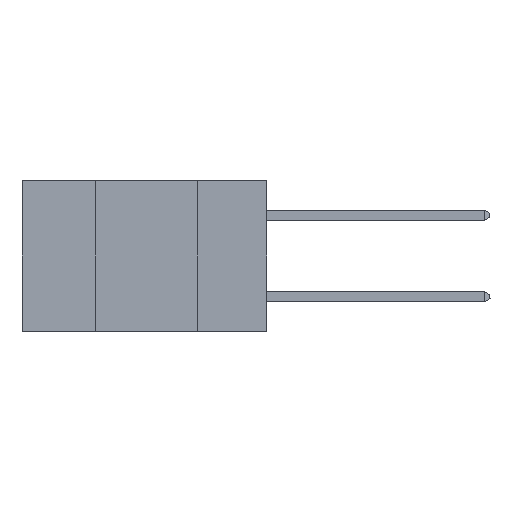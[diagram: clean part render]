
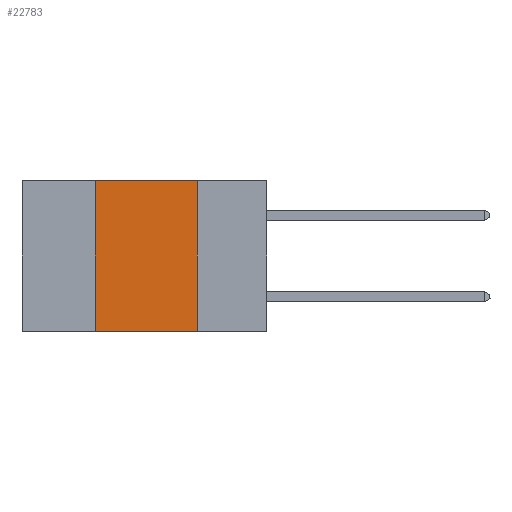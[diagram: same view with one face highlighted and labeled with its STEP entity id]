
A CAD part, left-side view. The second image highlights one B-rep face of the part: STEP entity #22783.
In plain terms, the highlighted planar face has unit normal (-1, 0, 0).
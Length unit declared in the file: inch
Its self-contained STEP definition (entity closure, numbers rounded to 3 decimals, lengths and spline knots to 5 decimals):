
#931 = VECTOR ( 'NONE', #15726, 39.37008 ) ;
#1160 = CARTESIAN_POINT ( 'NONE',  ( 0., 0.6, 0. ) ) ;
#2060 = LINE ( 'NONE', #25381, #29526 ) ;
#2293 = AXIS2_PLACEMENT_3D ( 'NONE', #1160, #17286, #24506 ) ;
#3103 = ORIENTED_EDGE ( 'NONE', *, *, #6593, .F. ) ;
#3889 = VERTEX_POINT ( 'NONE', #20650 ) ;
#4140 = CARTESIAN_POINT ( 'NONE',  ( 0., 0.42, 0. ) ) ;
#5482 = ORIENTED_EDGE ( 'NONE', *, *, #19721, .F. ) ;
#6108 = DIRECTION ( 'NONE',  ( 0., 0., -1. ) ) ;
#6310 = CARTESIAN_POINT ( 'NONE',  ( 0., 0.17, 0. ) ) ;
#6593 = EDGE_CURVE ( 'NONE', #18801, #10510, #7084, .T. ) ;
#7084 = LINE ( 'NONE', #4140, #931 ) ;
#7153 = CARTESIAN_POINT ( 'NONE',  ( 0., 0.42, -0.37 ) ) ;
#7213 = VECTOR ( 'NONE', #6108, 39.37008 ) ;
#10195 = ORIENTED_EDGE ( 'NONE', *, *, #24484, .T. ) ;
#10510 = VERTEX_POINT ( 'NONE', #27622 ) ;
#11272 = EDGE_LOOP ( 'NONE', ( #5482, #27780, #3103, #10195 ) ) ;
#11521 = DIRECTION ( 'NONE',  ( 0., -1., 0. ) ) ;
#14972 = PLANE ( 'NONE',  #2293 ) ;
#15726 = DIRECTION ( 'NONE',  ( 0., 0., 1. ) ) ;
#16009 = LINE ( 'NONE', #28918, #25049 ) ;
#17286 = DIRECTION ( 'NONE',  ( 1., 0., 0. ) ) ;
#18801 = VERTEX_POINT ( 'NONE', #7153 ) ;
#19678 = EDGE_CURVE ( 'NONE', #10510, #20355, #16009, .T. ) ;
#19721 = EDGE_CURVE ( 'NONE', #20355, #3889, #24591, .T. ) ;
#20355 = VERTEX_POINT ( 'NONE', #20448 ) ;
#20448 = CARTESIAN_POINT ( 'NONE',  ( 0., 0.17, 0. ) ) ;
#20650 = CARTESIAN_POINT ( 'NONE',  ( 0., 0.17, -0.37 ) ) ;
#22783 = ADVANCED_FACE ( 'NONE', ( #27465 ), #14972, .F. ) ;
#24484 = EDGE_CURVE ( 'NONE', #18801, #3889, #2060, .T. ) ;
#24506 = DIRECTION ( 'NONE',  ( 0., 0., -1. ) ) ;
#24591 = LINE ( 'NONE', #6310, #7213 ) ;
#25049 = VECTOR ( 'NONE', #26703, 39.37008 ) ;
#25381 = CARTESIAN_POINT ( 'NONE',  ( 0., 0.6, -0.37 ) ) ;
#26703 = DIRECTION ( 'NONE',  ( 0., -1., 0. ) ) ;
#27465 = FACE_OUTER_BOUND ( 'NONE', #11272, .T. ) ;
#27622 = CARTESIAN_POINT ( 'NONE',  ( 0., 0.42, 0. ) ) ;
#27780 = ORIENTED_EDGE ( 'NONE', *, *, #19678, .F. ) ;
#28918 = CARTESIAN_POINT ( 'NONE',  ( 0., 0.6, 0. ) ) ;
#29526 = VECTOR ( 'NONE', #11521, 39.37008 ) ;
